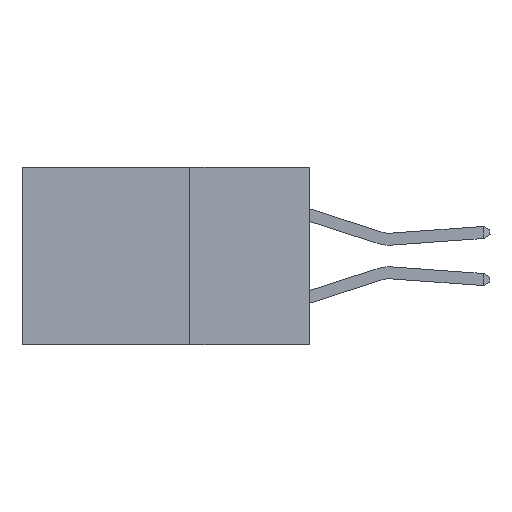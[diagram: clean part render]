
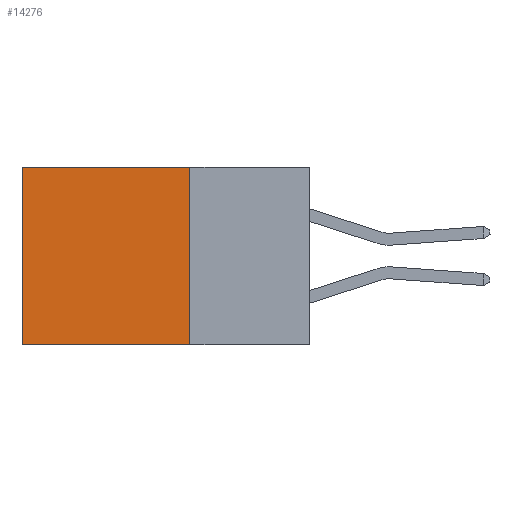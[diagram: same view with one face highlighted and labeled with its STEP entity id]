
A CAD part, left-side view. The second image highlights one B-rep face of the part: STEP entity #14276.
In plain terms, the highlighted planar face has unit normal (-1, 0, 0).
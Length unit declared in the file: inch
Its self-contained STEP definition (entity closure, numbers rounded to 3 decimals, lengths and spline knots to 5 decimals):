
#305 = CARTESIAN_POINT ( 'NONE',  ( 0.298, 0.6, 0. ) ) ;
#2288 = CARTESIAN_POINT ( 'NONE',  ( 0.298, 0.25, 0. ) ) ;
#4414 = DIRECTION ( 'NONE',  ( 0., 1., 0. ) ) ;
#5532 = VECTOR ( 'NONE', #4414, 39.37008 ) ;
#5643 = DIRECTION ( 'NONE',  ( 0., 0., -1. ) ) ;
#6364 = LINE ( 'NONE', #7069, #5532 ) ;
#7069 = CARTESIAN_POINT ( 'NONE',  ( 0.298, 0.25, -0.37 ) ) ;
#7587 = ORIENTED_EDGE ( 'NONE', *, *, #7771, .F. ) ;
#7617 = VERTEX_POINT ( 'NONE', #32108 ) ;
#7771 = EDGE_CURVE ( 'NONE', #30001, #7617, #6364, .T. ) ;
#8719 = VERTEX_POINT ( 'NONE', #28739 ) ;
#9168 = VECTOR ( 'NONE', #20691, 39.37008 ) ;
#9217 = EDGE_CURVE ( 'NONE', #8719, #30001, #29538, .T. ) ;
#12150 = DIRECTION ( 'NONE',  ( 0., 1., 0. ) ) ;
#12782 = PLANE ( 'NONE',  #22535 ) ;
#13178 = LINE ( 'NONE', #23670, #26014 ) ;
#14276 = ADVANCED_FACE ( 'NONE', ( #14845 ), #12782, .F. ) ;
#14845 = FACE_OUTER_BOUND ( 'NONE', #29016, .T. ) ;
#15351 = DIRECTION ( 'NONE',  ( 0., 0., -1. ) ) ;
#15542 = EDGE_CURVE ( 'NONE', #8719, #29599, #16388, .T. ) ;
#15560 = VECTOR ( 'NONE', #12150, 39.37008 ) ;
#16388 = LINE ( 'NONE', #17322, #15560 ) ;
#17322 = CARTESIAN_POINT ( 'NONE',  ( 0.298, 0.25, 0. ) ) ;
#18152 = CARTESIAN_POINT ( 'NONE',  ( 0.298, 0.25, 0. ) ) ;
#18605 = ORIENTED_EDGE ( 'NONE', *, *, #31602, .T. ) ;
#20691 = DIRECTION ( 'NONE',  ( 0., 0., -1. ) ) ;
#21100 = ORIENTED_EDGE ( 'NONE', *, *, #15542, .T. ) ;
#22535 = AXIS2_PLACEMENT_3D ( 'NONE', #2288, #30615, #15351 ) ;
#23670 = CARTESIAN_POINT ( 'NONE',  ( 0.298, 0.6, 0. ) ) ;
#26014 = VECTOR ( 'NONE', #5643, 39.37008 ) ;
#27711 = CARTESIAN_POINT ( 'NONE',  ( 0.298, 0.25, -0.37 ) ) ;
#28739 = CARTESIAN_POINT ( 'NONE',  ( 0.298, 0.25, 0. ) ) ;
#29016 = EDGE_LOOP ( 'NONE', ( #18605, #7587, #30466, #21100 ) ) ;
#29538 = LINE ( 'NONE', #18152, #9168 ) ;
#29599 = VERTEX_POINT ( 'NONE', #305 ) ;
#30001 = VERTEX_POINT ( 'NONE', #27711 ) ;
#30466 = ORIENTED_EDGE ( 'NONE', *, *, #9217, .F. ) ;
#30615 = DIRECTION ( 'NONE',  ( 1., 0., 0. ) ) ;
#31602 = EDGE_CURVE ( 'NONE', #29599, #7617, #13178, .T. ) ;
#32108 = CARTESIAN_POINT ( 'NONE',  ( 0.298, 0.6, -0.37 ) ) ;
